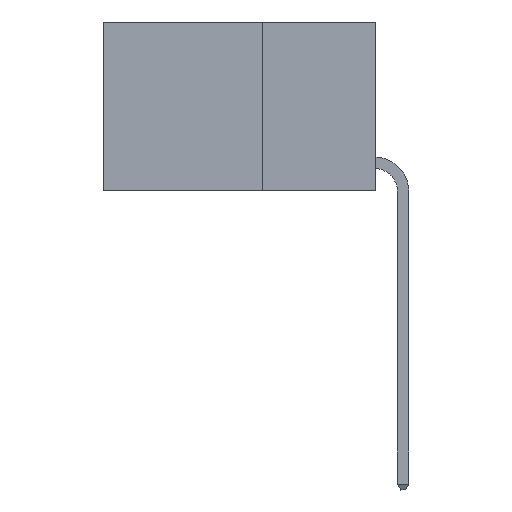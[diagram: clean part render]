
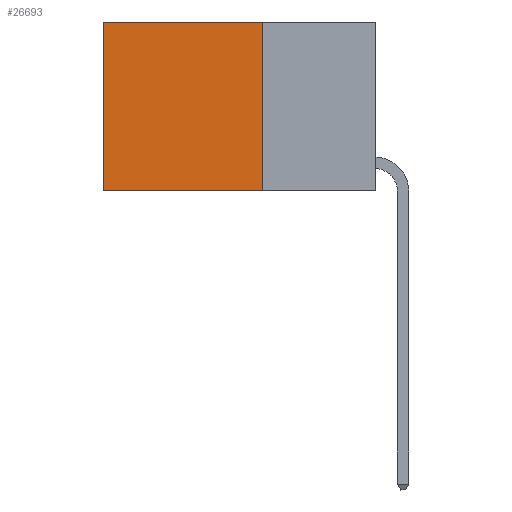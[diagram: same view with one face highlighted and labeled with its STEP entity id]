
A CAD part, left-side view. The second image highlights one B-rep face of the part: STEP entity #26693.
In plain terms, the highlighted planar face has unit normal (-1, 0, 0).
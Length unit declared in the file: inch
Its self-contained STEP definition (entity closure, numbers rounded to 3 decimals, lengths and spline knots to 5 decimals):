
#900 = DIRECTION ( 'NONE',  ( 1., 0., 0. ) ) ;
#1770 = VECTOR ( 'NONE', #11759, 39.37008 ) ;
#1827 = CARTESIAN_POINT ( 'NONE',  ( 0.2625, 0.6, 0. ) ) ;
#2793 = ORIENTED_EDGE ( 'NONE', *, *, #7905, .T. ) ;
#3636 = CARTESIAN_POINT ( 'NONE',  ( 0.2625, 0.25, 0. ) ) ;
#3826 = EDGE_LOOP ( 'NONE', ( #9225, #6421, #16829, #2793 ) ) ;
#4756 = LINE ( 'NONE', #14018, #1770 ) ;
#5329 = FACE_OUTER_BOUND ( 'NONE', #3826, .T. ) ;
#6417 = EDGE_CURVE ( 'NONE', #19612, #7694, #15522, .T. ) ;
#6421 = ORIENTED_EDGE ( 'NONE', *, *, #24812, .F. ) ;
#6677 = LINE ( 'NONE', #11228, #12972 ) ;
#7694 = VERTEX_POINT ( 'NONE', #27060 ) ;
#7905 = EDGE_CURVE ( 'NONE', #15895, #19612, #12750, .T. ) ;
#9225 = ORIENTED_EDGE ( 'NONE', *, *, #6417, .T. ) ;
#10173 = DIRECTION ( 'NONE',  ( 0., 0., -1. ) ) ;
#10323 = DIRECTION ( 'NONE',  ( 0., 1., 0. ) ) ;
#11228 = CARTESIAN_POINT ( 'NONE',  ( 0.2625, 0.25, 0. ) ) ;
#11759 = DIRECTION ( 'NONE',  ( 0., 1., 0. ) ) ;
#12450 = CARTESIAN_POINT ( 'NONE',  ( 0.2625, 0.25, 0. ) ) ;
#12750 = LINE ( 'NONE', #3636, #18815 ) ;
#12972 = VECTOR ( 'NONE', #17629, 39.37008 ) ;
#14018 = CARTESIAN_POINT ( 'NONE',  ( 0.2625, 0.25, -0.37 ) ) ;
#14372 = EDGE_CURVE ( 'NONE', #15895, #20197, #6677, .T. ) ;
#15522 = LINE ( 'NONE', #1827, #25360 ) ;
#15895 = VERTEX_POINT ( 'NONE', #22014 ) ;
#16829 = ORIENTED_EDGE ( 'NONE', *, *, #14372, .F. ) ;
#17629 = DIRECTION ( 'NONE',  ( 0., 0., -1. ) ) ;
#18556 = CARTESIAN_POINT ( 'NONE',  ( 0.2625, 0.25, -0.37 ) ) ;
#18815 = VECTOR ( 'NONE', #10323, 39.37008 ) ;
#19612 = VERTEX_POINT ( 'NONE', #28425 ) ;
#20197 = VERTEX_POINT ( 'NONE', #18556 ) ;
#20761 = AXIS2_PLACEMENT_3D ( 'NONE', #12450, #900, #10173 ) ;
#22014 = CARTESIAN_POINT ( 'NONE',  ( 0.2625, 0.25, 0. ) ) ;
#23963 = PLANE ( 'NONE',  #20761 ) ;
#24743 = DIRECTION ( 'NONE',  ( 0., 0., -1. ) ) ;
#24812 = EDGE_CURVE ( 'NONE', #20197, #7694, #4756, .T. ) ;
#25360 = VECTOR ( 'NONE', #24743, 39.37008 ) ;
#26693 = ADVANCED_FACE ( 'NONE', ( #5329 ), #23963, .F. ) ;
#27060 = CARTESIAN_POINT ( 'NONE',  ( 0.2625, 0.6, -0.37 ) ) ;
#28425 = CARTESIAN_POINT ( 'NONE',  ( 0.2625, 0.6, 0. ) ) ;
